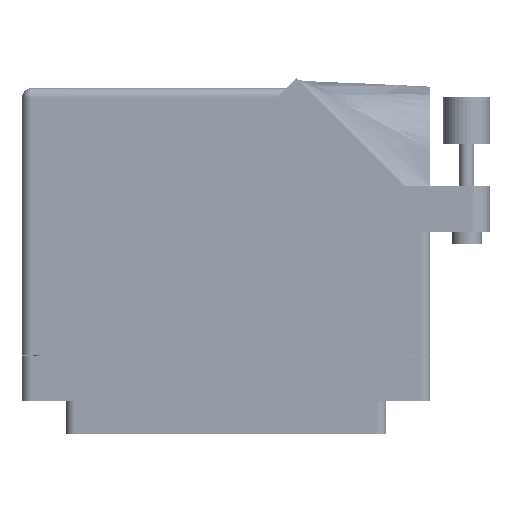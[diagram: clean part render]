
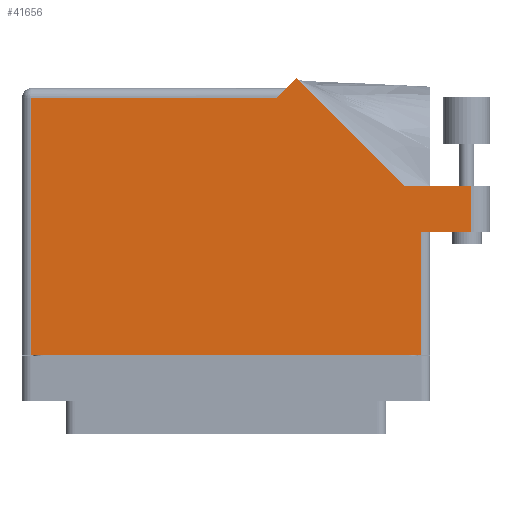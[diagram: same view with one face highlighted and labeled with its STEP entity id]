
A CAD part, front view. The second image highlights one B-rep face of the part: STEP entity #41656.
In plain terms, the highlighted face is planar.
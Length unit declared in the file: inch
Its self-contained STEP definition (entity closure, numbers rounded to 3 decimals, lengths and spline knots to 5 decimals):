
#1319 = EDGE_CURVE ( 'NONE', #71479, #24185, #3531, .T. ) ;
#3470 = LINE ( 'NONE', #32804, #27454 ) ;
#3531 = LINE ( 'NONE', #49153, #19536 ) ;
#3871 = DIRECTION ( 'NONE',  ( -1., 0., 0. ) ) ;
#5240 = EDGE_CURVE ( 'NONE', #68161, #42487, #12089, .T. ) ;
#6496 = DIRECTION ( 'NONE',  ( 1., 0., 0. ) ) ;
#8083 = CARTESIAN_POINT ( 'NONE',  ( 0.46971, 1.74571, 0.617 ) ) ;
#9798 = CARTESIAN_POINT ( 'NONE',  ( 1.19342, 1.022, 0.617 ) ) ;
#12089 = LINE ( 'NONE', #25679, #21895 ) ;
#12495 = VECTOR ( 'NONE', #35870, 39.37008 ) ;
#16481 = CARTESIAN_POINT ( 'NONE',  ( 1.297, 0.715, 0.617 ) ) ;
#16567 = VERTEX_POINT ( 'NONE', #62527 ) ;
#17474 = CARTESIAN_POINT ( 'NONE',  ( -1.359, -0.1, 0.617 ) ) ;
#18933 = CARTESIAN_POINT ( 'NONE',  ( 0.337, 1.613, 0.617 ) ) ;
#19536 = VECTOR ( 'NONE', #31355, 39.37008 ) ;
#20033 = ORIENTED_EDGE ( 'NONE', *, *, #63467, .T. ) ;
#20043 = ORIENTED_EDGE ( 'NONE', *, *, #1319, .T. ) ;
#21050 = DIRECTION ( 'NONE',  ( 0., 1., 0. ) ) ;
#21895 = VECTOR ( 'NONE', #53966, 39.37008 ) ;
#23381 = EDGE_CURVE ( 'NONE', #24185, #53829, #3470, .T. ) ;
#24185 = VERTEX_POINT ( 'NONE', #63321 ) ;
#24760 = PLANE ( 'NONE',  #51236 ) ;
#25406 = ORIENTED_EDGE ( 'NONE', *, *, #23381, .T. ) ;
#25679 = CARTESIAN_POINT ( 'NONE',  ( 0.399, 1.675, 0.617 ) ) ;
#27332 = VERTEX_POINT ( 'NONE', #33064 ) ;
#27454 = VECTOR ( 'NONE', #21050, 39.37008 ) ;
#27833 = EDGE_LOOP ( 'NONE', ( #20043, #25406, #38633, #46696, #70773, #20033, #64943, #70039, #58180 ) ) ;
#30007 = CARTESIAN_POINT ( 'NONE',  ( 1.297, 0.715, 0.617 ) ) ;
#30565 = LINE ( 'NONE', #59669, #55680 ) ;
#30980 = DIRECTION ( 'NONE',  ( 0., 0., -1. ) ) ;
#31021 = CARTESIAN_POINT ( 'NONE',  ( -1.297, 1.613, 0.617 ) ) ;
#31355 = DIRECTION ( 'NONE',  ( 1., 0., 0. ) ) ;
#32804 = CARTESIAN_POINT ( 'NONE',  ( 1.634, 1.022, 0.617 ) ) ;
#33064 = CARTESIAN_POINT ( 'NONE',  ( 1.19342, 1.022, 0.617 ) ) ;
#33606 = EDGE_CURVE ( 'NONE', #69335, #16567, #50945, .T. ) ;
#34880 = VECTOR ( 'NONE', #55783, 39.37008 ) ;
#35870 = DIRECTION ( 'NONE',  ( 0., 1., 0. ) ) ;
#36557 = CARTESIAN_POINT ( 'NONE',  ( -1.359, 1.675, 0.617 ) ) ;
#37544 = DIRECTION ( 'NONE',  ( -1., 0., 0. ) ) ;
#38633 = ORIENTED_EDGE ( 'NONE', *, *, #50050, .T. ) ;
#41656 = ADVANCED_FACE ( 'NONE', ( #63984 ), #24760, .F. ) ;
#42399 = LINE ( 'NONE', #17474, #69187 ) ;
#42487 = VERTEX_POINT ( 'NONE', #18933 ) ;
#43286 = EDGE_CURVE ( 'NONE', #16567, #61808, #42399, .T. ) ;
#46696 = ORIENTED_EDGE ( 'NONE', *, *, #53623, .T. ) ;
#49139 = EDGE_CURVE ( 'NONE', #61808, #71479, #60739, .T. ) ;
#49153 = CARTESIAN_POINT ( 'NONE',  ( 1.359, 0.715, 0.617 ) ) ;
#49727 = DIRECTION ( 'NONE',  ( -0.707, 0.707, 0. ) ) ;
#50050 = EDGE_CURVE ( 'NONE', #53829, #27332, #58903, .T. ) ;
#50945 = LINE ( 'NONE', #67743, #34880 ) ;
#51236 = AXIS2_PLACEMENT_3D ( 'NONE', #36557, #30980, #71003 ) ;
#53056 = CARTESIAN_POINT ( 'NONE',  ( 1.297, -0.1, 0.617 ) ) ;
#53623 = EDGE_CURVE ( 'NONE', #27332, #68161, #57415, .T. ) ;
#53829 = VERTEX_POINT ( 'NONE', #63156 ) ;
#53966 = DIRECTION ( 'NONE',  ( -0.707, -0.707, 0. ) ) ;
#55408 = VECTOR ( 'NONE', #3871, 39.37008 ) ;
#55680 = VECTOR ( 'NONE', #37544, 39.37008 ) ;
#55783 = DIRECTION ( 'NONE',  ( 0., -1., 0. ) ) ;
#57415 = LINE ( 'NONE', #9798, #62831 ) ;
#58180 = ORIENTED_EDGE ( 'NONE', *, *, #49139, .T. ) ;
#58903 = LINE ( 'NONE', #71491, #55408 ) ;
#59669 = CARTESIAN_POINT ( 'NONE',  ( -1.359, 1.613, 0.617 ) ) ;
#60739 = LINE ( 'NONE', #30007, #12495 ) ;
#61808 = VERTEX_POINT ( 'NONE', #53056 ) ;
#62527 = CARTESIAN_POINT ( 'NONE',  ( -1.297, -0.1, 0.617 ) ) ;
#62831 = VECTOR ( 'NONE', #49727, 39.37008 ) ;
#63156 = CARTESIAN_POINT ( 'NONE',  ( 1.634, 1.022, 0.617 ) ) ;
#63321 = CARTESIAN_POINT ( 'NONE',  ( 1.634, 0.715, 0.617 ) ) ;
#63467 = EDGE_CURVE ( 'NONE', #42487, #69335, #30565, .T. ) ;
#63984 = FACE_OUTER_BOUND ( 'NONE', #27833, .T. ) ;
#64943 = ORIENTED_EDGE ( 'NONE', *, *, #33606, .T. ) ;
#67743 = CARTESIAN_POINT ( 'NONE',  ( -1.297, -0.1, 0.617 ) ) ;
#68161 = VERTEX_POINT ( 'NONE', #8083 ) ;
#69187 = VECTOR ( 'NONE', #6496, 39.37008 ) ;
#69335 = VERTEX_POINT ( 'NONE', #31021 ) ;
#70039 = ORIENTED_EDGE ( 'NONE', *, *, #43286, .T. ) ;
#70773 = ORIENTED_EDGE ( 'NONE', *, *, #5240, .T. ) ;
#71003 = DIRECTION ( 'NONE',  ( -1., 0., 0. ) ) ;
#71479 = VERTEX_POINT ( 'NONE', #16481 ) ;
#71491 = CARTESIAN_POINT ( 'NONE',  ( 1.759, 1.022, 0.617 ) ) ;
